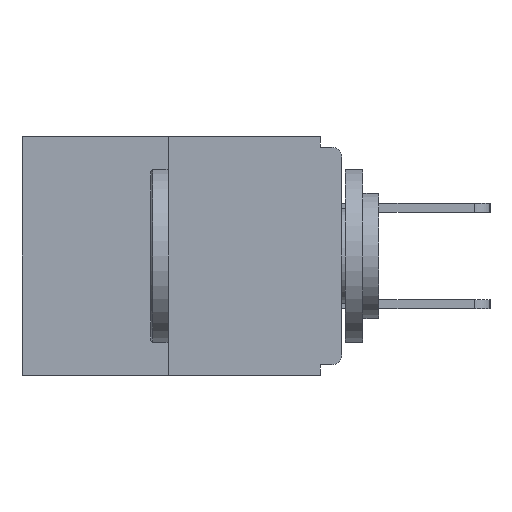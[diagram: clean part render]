
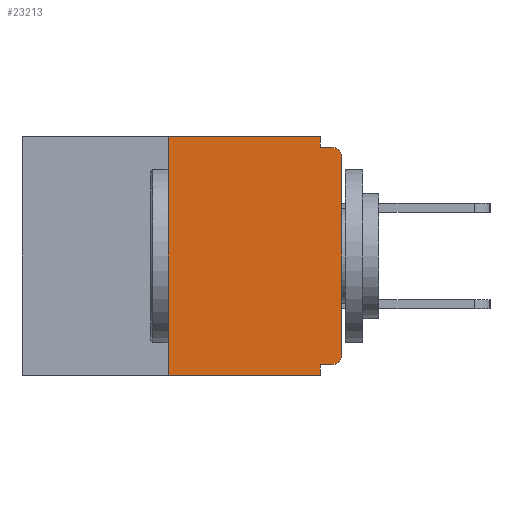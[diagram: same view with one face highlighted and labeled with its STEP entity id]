
A CAD part, left-side view. The second image highlights one B-rep face of the part: STEP entity #23213.
In plain terms, the highlighted planar face has unit normal (-1, 0, 0).
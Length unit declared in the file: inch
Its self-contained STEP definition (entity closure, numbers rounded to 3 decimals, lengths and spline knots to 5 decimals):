
#647 = DIRECTION ( 'NONE',  ( 0., 0., 1. ) ) ;
#999 = VECTOR ( 'NONE', #24981, 39.37008 ) ;
#1216 = DIRECTION ( 'NONE',  ( 0., -1., 0. ) ) ;
#1570 = CARTESIAN_POINT ( 'NONE',  ( 0., 0.015, -0.03 ) ) ;
#2061 = CARTESIAN_POINT ( 'NONE',  ( 0., 0., -0.03 ) ) ;
#2392 = CARTESIAN_POINT ( 'NONE',  ( 0., 0.015, -0.015 ) ) ;
#2429 = VERTEX_POINT ( 'NONE', #15764 ) ;
#3448 = VECTOR ( 'NONE', #647, 39.37008 ) ;
#3544 = CARTESIAN_POINT ( 'NONE',  ( 0., 0.25, -0.343 ) ) ;
#3609 = VERTEX_POINT ( 'NONE', #2392 ) ;
#4107 = LINE ( 'NONE', #26354, #9903 ) ;
#4187 = CARTESIAN_POINT ( 'NONE',  ( 0., 0.46, 0. ) ) ;
#4239 = LINE ( 'NONE', #12982, #3448 ) ;
#4286 = DIRECTION ( 'NONE',  ( 0., 0., -1. ) ) ;
#4295 = DIRECTION ( 'NONE',  ( 1., 0., 0. ) ) ;
#4302 = EDGE_CURVE ( 'NONE', #20597, #12241, #4107, .T. ) ;
#4723 = DIRECTION ( 'NONE',  ( 0., 0., -1. ) ) ;
#5981 = EDGE_CURVE ( 'NONE', #2429, #8419, #24871, .T. ) ;
#6336 = DIRECTION ( 'NONE',  ( 0., 0., 1. ) ) ;
#6972 = DIRECTION ( 'NONE',  ( -1., 0., 0. ) ) ;
#7558 = CARTESIAN_POINT ( 'NONE',  ( 0., 0.46, -0.343 ) ) ;
#7724 = VECTOR ( 'NONE', #1216, 39.37008 ) ;
#7786 = VECTOR ( 'NONE', #4723, 39.37008 ) ;
#8112 = VERTEX_POINT ( 'NONE', #3544 ) ;
#8419 = VERTEX_POINT ( 'NONE', #12585 ) ;
#8434 = ORIENTED_EDGE ( 'NONE', *, *, #11022, .T. ) ;
#8745 = EDGE_CURVE ( 'NONE', #8112, #20597, #27428, .T. ) ;
#9041 = ORIENTED_EDGE ( 'NONE', *, *, #5981, .F. ) ;
#9473 = CARTESIAN_POINT ( 'NONE',  ( 0., 0.031, 0. ) ) ;
#9750 = LINE ( 'NONE', #7558, #24108 ) ;
#9903 = VECTOR ( 'NONE', #24298, 39.37008 ) ;
#10345 = AXIS2_PLACEMENT_3D ( 'NONE', #13744, #16028, #31060 ) ;
#11022 = EDGE_CURVE ( 'NONE', #28086, #3609, #28435, .T. ) ;
#11854 = LINE ( 'NONE', #29598, #999 ) ;
#12091 = CIRCLE ( 'NONE', #10345, 0.015 ) ;
#12241 = VERTEX_POINT ( 'NONE', #27022 ) ;
#12585 = CARTESIAN_POINT ( 'NONE',  ( 0., 0.031, -0.328 ) ) ;
#12982 = CARTESIAN_POINT ( 'NONE',  ( 0., 0., 0. ) ) ;
#13744 = CARTESIAN_POINT ( 'NONE',  ( 0., 0.015, -0.313 ) ) ;
#14283 = ORIENTED_EDGE ( 'NONE', *, *, #26602, .T. ) ;
#14832 = AXIS2_PLACEMENT_3D ( 'NONE', #1570, #6972, #4286 ) ;
#15764 = CARTESIAN_POINT ( 'NONE',  ( 0., 0.015, -0.328 ) ) ;
#15894 = LINE ( 'NONE', #9473, #7786 ) ;
#16028 = DIRECTION ( 'NONE',  ( -1., 0., 0. ) ) ;
#16054 = EDGE_CURVE ( 'NONE', #8419, #29516, #11854, .T. ) ;
#16230 = EDGE_LOOP ( 'NONE', ( #24424, #31516, #14283, #16993, #9041, #24849, #22719, #8434, #16974, #19719 ) ) ;
#16974 = ORIENTED_EDGE ( 'NONE', *, *, #27497, .F. ) ;
#16993 = ORIENTED_EDGE ( 'NONE', *, *, #16054, .F. ) ;
#17346 = VERTEX_POINT ( 'NONE', #29591 ) ;
#19719 = ORIENTED_EDGE ( 'NONE', *, *, #21282, .F. ) ;
#20597 = VERTEX_POINT ( 'NONE', #30997 ) ;
#21196 = FACE_OUTER_BOUND ( 'NONE', #16230, .T. ) ;
#21282 = EDGE_CURVE ( 'NONE', #12241, #17346, #15894, .T. ) ;
#22402 = CARTESIAN_POINT ( 'NONE',  ( 0., 0., -0.328 ) ) ;
#22413 = VECTOR ( 'NONE', #6336, 39.37008 ) ;
#22719 = ORIENTED_EDGE ( 'NONE', *, *, #27837, .T. ) ;
#23135 = CARTESIAN_POINT ( 'NONE',  ( 0., 0.031, -0.343 ) ) ;
#23213 = ADVANCED_FACE ( 'NONE', ( #21196 ), #23882, .F. ) ;
#23882 = PLANE ( 'NONE',  #26366 ) ;
#24010 = LINE ( 'NONE', #28349, #7724 ) ;
#24108 = VECTOR ( 'NONE', #25092, 39.37008 ) ;
#24298 = DIRECTION ( 'NONE',  ( 0., -1., 0. ) ) ;
#24424 = ORIENTED_EDGE ( 'NONE', *, *, #4302, .F. ) ;
#24849 = ORIENTED_EDGE ( 'NONE', *, *, #30829, .T. ) ;
#24871 = LINE ( 'NONE', #22402, #26440 ) ;
#24981 = DIRECTION ( 'NONE',  ( 0., 0., -1. ) ) ;
#25092 = DIRECTION ( 'NONE',  ( 0., -1., 0. ) ) ;
#26354 = CARTESIAN_POINT ( 'NONE',  ( 0., 0.46, 0. ) ) ;
#26362 = DIRECTION ( 'NONE',  ( 0., 0., -1. ) ) ;
#26366 = AXIS2_PLACEMENT_3D ( 'NONE', #4187, #4295, #26362 ) ;
#26440 = VECTOR ( 'NONE', #27474, 39.37008 ) ;
#26602 = EDGE_CURVE ( 'NONE', #8112, #29516, #9750, .T. ) ;
#27022 = CARTESIAN_POINT ( 'NONE',  ( 0., 0.031, 0. ) ) ;
#27290 = CARTESIAN_POINT ( 'NONE',  ( 0., 0., -0.313 ) ) ;
#27428 = LINE ( 'NONE', #31138, #22413 ) ;
#27474 = DIRECTION ( 'NONE',  ( 0., 1., 0. ) ) ;
#27497 = EDGE_CURVE ( 'NONE', #17346, #3609, #24010, .T. ) ;
#27837 = EDGE_CURVE ( 'NONE', #29683, #28086, #4239, .T. ) ;
#28086 = VERTEX_POINT ( 'NONE', #2061 ) ;
#28349 = CARTESIAN_POINT ( 'NONE',  ( 0., 0., -0.015 ) ) ;
#28435 = CIRCLE ( 'NONE', #14832, 0.015 ) ;
#29516 = VERTEX_POINT ( 'NONE', #23135 ) ;
#29591 = CARTESIAN_POINT ( 'NONE',  ( 0., 0.031, -0.015 ) ) ;
#29598 = CARTESIAN_POINT ( 'NONE',  ( 0., 0.031, -0.343 ) ) ;
#29683 = VERTEX_POINT ( 'NONE', #27290 ) ;
#30829 = EDGE_CURVE ( 'NONE', #2429, #29683, #12091, .T. ) ;
#30997 = CARTESIAN_POINT ( 'NONE',  ( 0., 0.25, 0. ) ) ;
#31060 = DIRECTION ( 'NONE',  ( 0., 0., -1. ) ) ;
#31138 = CARTESIAN_POINT ( 'NONE',  ( 0., 0.25, 0. ) ) ;
#31516 = ORIENTED_EDGE ( 'NONE', *, *, #8745, .F. ) ;
